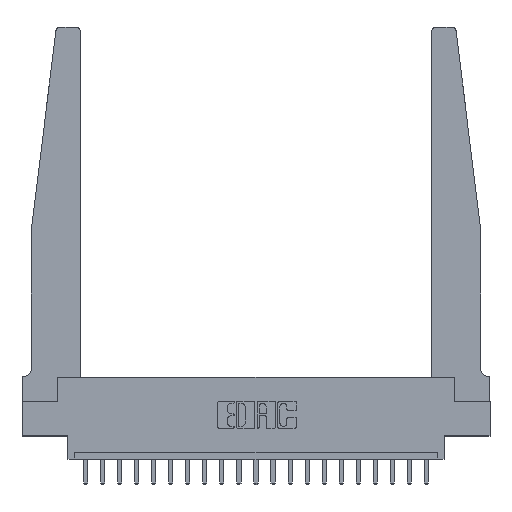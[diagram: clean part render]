
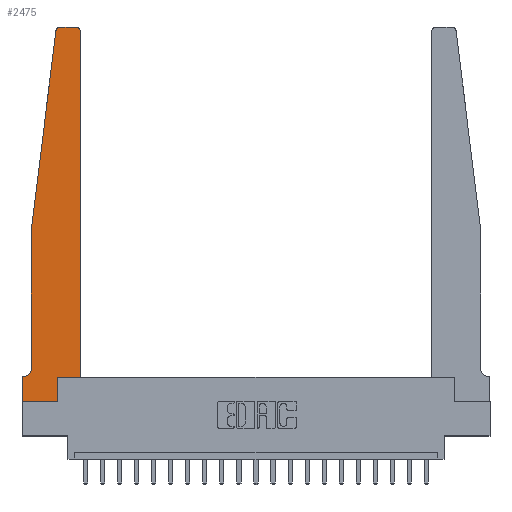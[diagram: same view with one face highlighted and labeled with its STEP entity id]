
A CAD part, top view. The second image highlights one B-rep face of the part: STEP entity #2475.
In plain terms, the highlighted planar face has unit normal (0, 0, 1).
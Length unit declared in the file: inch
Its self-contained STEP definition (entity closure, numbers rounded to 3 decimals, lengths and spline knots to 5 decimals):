
#133 = DIRECTION ( 'NONE',  ( 0., 0., 1. ) ) ;
#244 = AXIS2_PLACEMENT_3D ( 'NONE', #8324, #133, #3495 ) ;
#271 = VERTEX_POINT ( 'NONE', #6402 ) ;
#488 = AXIS2_PLACEMENT_3D ( 'NONE', #1465, #17514, #17938 ) ;
#692 = CIRCLE ( 'NONE', #9650, 0.03 ) ;
#903 = VERTEX_POINT ( 'NONE', #11260 ) ;
#949 = EDGE_CURVE ( 'NONE', #10097, #8620, #7925, .T. ) ;
#1465 = CARTESIAN_POINT ( 'NONE',  ( 0.015, 0.2375, 0.37 ) ) ;
#1510 = CARTESIAN_POINT ( 'NONE',  ( 0., 0., 0.37 ) ) ;
#1710 = VERTEX_POINT ( 'NONE', #14718 ) ;
#1757 = FACE_OUTER_BOUND ( 'NONE', #18010, .T. ) ;
#1879 = LINE ( 'NONE', #13390, #3057 ) ;
#1975 = DIRECTION ( 'NONE',  ( 0., 0., 1. ) ) ;
#2041 = VERTEX_POINT ( 'NONE', #16490 ) ;
#2100 = CARTESIAN_POINT ( 'NONE',  ( 0.065, 0.1875, 0.37 ) ) ;
#2475 = ADVANCED_FACE ( 'NONE', ( #1757 ), #19852, .T. ) ;
#2514 = VERTEX_POINT ( 'NONE', #2756 ) ;
#2633 = EDGE_CURVE ( 'NONE', #2514, #903, #8067, .T. ) ;
#2756 = CARTESIAN_POINT ( 'NONE',  ( 0.395, 2.75, 0.37 ) ) ;
#2885 = DIRECTION ( 'NONE',  ( 1., 0., 0. ) ) ;
#3057 = VECTOR ( 'NONE', #7065, 39.37008 ) ;
#3452 = DIRECTION ( 'NONE',  ( 0., -1., 0. ) ) ;
#3495 = DIRECTION ( 'NONE',  ( 1., 0., 0. ) ) ;
#4075 = VERTEX_POINT ( 'NONE', #19167 ) ;
#4249 = DIRECTION ( 'NONE',  ( 1., 0., 0. ) ) ;
#4445 = VECTOR ( 'NONE', #4249, 39.37008 ) ;
#4978 = CARTESIAN_POINT ( 'NONE',  ( 0.395, 2.72, 0.37 ) ) ;
#5092 = DIRECTION ( 'NONE',  ( 1., 0., 0. ) ) ;
#5166 = LINE ( 'NONE', #16544, #7000 ) ;
#5407 = CARTESIAN_POINT ( 'NONE',  ( 0.065, 0.2375, 0.37 ) ) ;
#5616 = ORIENTED_EDGE ( 'NONE', *, *, #15542, .T. ) ;
#5841 = VERTEX_POINT ( 'NONE', #9339 ) ;
#6033 = EDGE_CURVE ( 'NONE', #4075, #2041, #1879, .T. ) ;
#6059 = VECTOR ( 'NONE', #8615, 39.37008 ) ;
#6102 = AXIS2_PLACEMENT_3D ( 'NONE', #20291, #1975, #10155 ) ;
#6402 = CARTESIAN_POINT ( 'NONE',  ( 0.2605, 0.18, 0.37 ) ) ;
#6621 = CARTESIAN_POINT ( 'NONE',  ( 0.065, 1.25, 0.37 ) ) ;
#6863 = VECTOR ( 'NONE', #20171, 39.37008 ) ;
#7000 = VECTOR ( 'NONE', #3452, 39.37008 ) ;
#7065 = DIRECTION ( 'NONE',  ( 0., 1., 0. ) ) ;
#7422 = CARTESIAN_POINT ( 'NONE',  ( 0., 0.1875, 0.37 ) ) ;
#7925 = LINE ( 'NONE', #14140, #15683 ) ;
#8067 = LINE ( 'NONE', #11414, #8482 ) ;
#8324 = CARTESIAN_POINT ( 'NONE',  ( 0., 0.1875, 0.37 ) ) ;
#8482 = VECTOR ( 'NONE', #16237, 39.37008 ) ;
#8519 = DIRECTION ( 'NONE',  ( 0., 0., 1. ) ) ;
#8531 = LINE ( 'NONE', #6621, #6863 ) ;
#8615 = DIRECTION ( 'NONE',  ( 0., 1., 0. ) ) ;
#8620 = VERTEX_POINT ( 'NONE', #1510 ) ;
#8899 = ORIENTED_EDGE ( 'NONE', *, *, #13324, .T. ) ;
#9068 = LINE ( 'NONE', #20516, #4445 ) ;
#9339 = CARTESIAN_POINT ( 'NONE',  ( 0.2605, 0., 0.37 ) ) ;
#9498 = ORIENTED_EDGE ( 'NONE', *, *, #6033, .T. ) ;
#9650 = AXIS2_PLACEMENT_3D ( 'NONE', #4978, #8519, #5092 ) ;
#9803 = CARTESIAN_POINT ( 'NONE',  ( 0.2605, 0.18, 0.37 ) ) ;
#9902 = ORIENTED_EDGE ( 'NONE', *, *, #19414, .T. ) ;
#9917 = VERTEX_POINT ( 'NONE', #5407 ) ;
#10097 = VERTEX_POINT ( 'NONE', #7422 ) ;
#10155 = DIRECTION ( 'NONE',  ( 1., 0., 0. ) ) ;
#10925 = CARTESIAN_POINT ( 'NONE',  ( 0.24675, 2.72367, 0.37 ) ) ;
#10981 = ORIENTED_EDGE ( 'NONE', *, *, #13624, .T. ) ;
#11042 = CARTESIAN_POINT ( 'NONE',  ( 0.425, 0.18, 0.37 ) ) ;
#11260 = CARTESIAN_POINT ( 'NONE',  ( 0.27653, 2.75, 0.37 ) ) ;
#11304 = ORIENTED_EDGE ( 'NONE', *, *, #11593, .T. ) ;
#11365 = ORIENTED_EDGE ( 'NONE', *, *, #16770, .T. ) ;
#11391 = EDGE_CURVE ( 'NONE', #20566, #9917, #5166, .T. ) ;
#11414 = CARTESIAN_POINT ( 'NONE',  ( 0.25, 2.75, 0.37 ) ) ;
#11593 = EDGE_CURVE ( 'NONE', #9917, #1710, #19077, .T. ) ;
#12476 = ORIENTED_EDGE ( 'NONE', *, *, #2633, .T. ) ;
#13170 = ORIENTED_EDGE ( 'NONE', *, *, #16477, .T. ) ;
#13324 = EDGE_CURVE ( 'NONE', #1710, #10097, #13377, .T. ) ;
#13377 = LINE ( 'NONE', #2100, #20231 ) ;
#13390 = CARTESIAN_POINT ( 'NONE',  ( 0.425, 0.18, 0.37 ) ) ;
#13440 = LINE ( 'NONE', #9803, #6059 ) ;
#13624 = EDGE_CURVE ( 'NONE', #2041, #2514, #692, .T. ) ;
#13924 = VECTOR ( 'NONE', #2885, 39.37008 ) ;
#14140 = CARTESIAN_POINT ( 'NONE',  ( 0., 0., 0.37 ) ) ;
#14648 = CARTESIAN_POINT ( 'NONE',  ( 0.065, 1.25, 0.37 ) ) ;
#14718 = CARTESIAN_POINT ( 'NONE',  ( 0.015, 0.1875, 0.37 ) ) ;
#14965 = CIRCLE ( 'NONE', #6102, 0.03 ) ;
#15015 = ORIENTED_EDGE ( 'NONE', *, *, #19175, .T. ) ;
#15542 = EDGE_CURVE ( 'NONE', #5841, #271, #13440, .T. ) ;
#15683 = VECTOR ( 'NONE', #20864, 39.37008 ) ;
#15718 = ORIENTED_EDGE ( 'NONE', *, *, #11391, .T. ) ;
#16237 = DIRECTION ( 'NONE',  ( -1., 0., 0. ) ) ;
#16477 = EDGE_CURVE ( 'NONE', #271, #4075, #19237, .T. ) ;
#16490 = CARTESIAN_POINT ( 'NONE',  ( 0.425, 2.72, 0.37 ) ) ;
#16523 = VERTEX_POINT ( 'NONE', #10925 ) ;
#16544 = CARTESIAN_POINT ( 'NONE',  ( 0.065, 1.25, 0.37 ) ) ;
#16597 = DIRECTION ( 'NONE',  ( -1., 0., 0. ) ) ;
#16770 = EDGE_CURVE ( 'NONE', #903, #16523, #14965, .T. ) ;
#17514 = DIRECTION ( 'NONE',  ( 0., 0., -1. ) ) ;
#17938 = DIRECTION ( 'NONE',  ( -1., 0., 0. ) ) ;
#18010 = EDGE_LOOP ( 'NONE', ( #12476, #11365, #9902, #15718, #11304, #8899, #18565, #15015, #5616, #13170, #9498, #10981 ) ) ;
#18565 = ORIENTED_EDGE ( 'NONE', *, *, #949, .T. ) ;
#19077 = CIRCLE ( 'NONE', #488, 0.05 ) ;
#19167 = CARTESIAN_POINT ( 'NONE',  ( 0.425, 0.18, 0.37 ) ) ;
#19175 = EDGE_CURVE ( 'NONE', #8620, #5841, #9068, .T. ) ;
#19237 = LINE ( 'NONE', #11042, #13924 ) ;
#19414 = EDGE_CURVE ( 'NONE', #16523, #20566, #8531, .T. ) ;
#19852 = PLANE ( 'NONE',  #244 ) ;
#20171 = DIRECTION ( 'NONE',  ( -0.122, -0.992, 0. ) ) ;
#20231 = VECTOR ( 'NONE', #16597, 39.37008 ) ;
#20291 = CARTESIAN_POINT ( 'NONE',  ( 0.27653, 2.72, 0.37 ) ) ;
#20516 = CARTESIAN_POINT ( 'NONE',  ( 0., 0., 0.37 ) ) ;
#20566 = VERTEX_POINT ( 'NONE', #14648 ) ;
#20864 = DIRECTION ( 'NONE',  ( 0., -1., 0. ) ) ;
